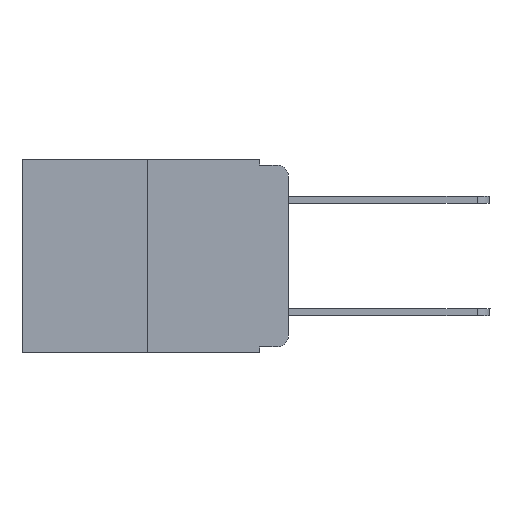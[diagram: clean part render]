
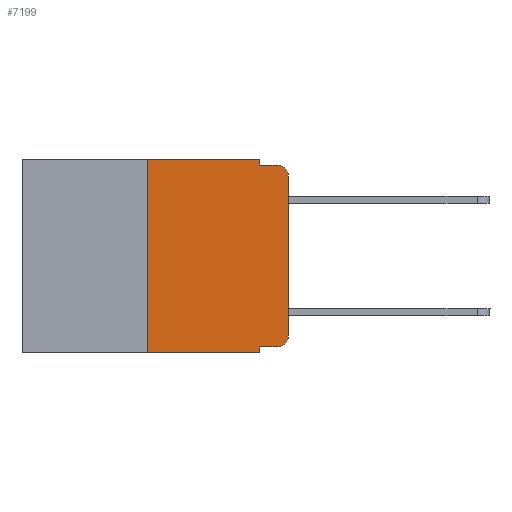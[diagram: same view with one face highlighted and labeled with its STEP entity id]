
A CAD part, left-side view. The second image highlights one B-rep face of the part: STEP entity #7199.
In plain terms, the highlighted planar face has unit normal (-1, 0, 0).
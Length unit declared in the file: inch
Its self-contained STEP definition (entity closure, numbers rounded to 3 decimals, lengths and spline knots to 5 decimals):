
#100 = CARTESIAN_POINT ( 'NONE',  ( 0., 0.25, 0. ) ) ;
#232 = VERTEX_POINT ( 'NONE', #6437 ) ;
#743 = DIRECTION ( 'NONE',  ( 0., 0., -1. ) ) ;
#809 = LINE ( 'NONE', #5505, #2120 ) ;
#894 = CARTESIAN_POINT ( 'NONE',  ( 0., 0.051, 0. ) ) ;
#1016 = DIRECTION ( 'NONE',  ( 0., 0., -1. ) ) ;
#1036 = CARTESIAN_POINT ( 'NONE',  ( 0., 0.051, 0. ) ) ;
#1127 = LINE ( 'NONE', #10622, #5782 ) ;
#1220 = AXIS2_PLACEMENT_3D ( 'NONE', #9701, #6009, #1016 ) ;
#1239 = DIRECTION ( 'NONE',  ( 0., 0., 1. ) ) ;
#1463 = VERTEX_POINT ( 'NONE', #8393 ) ;
#1633 = VECTOR ( 'NONE', #11658, 39.37008 ) ;
#1642 = CIRCLE ( 'NONE', #1220, 0.02 ) ;
#1655 = EDGE_CURVE ( 'NONE', #2808, #3309, #1127, .T. ) ;
#1686 = PLANE ( 'NONE',  #7245 ) ;
#1688 = ORIENTED_EDGE ( 'NONE', *, *, #10585, .F. ) ;
#1778 = LINE ( 'NONE', #8451, #8004 ) ;
#2067 = CARTESIAN_POINT ( 'NONE',  ( 0., 0., -0.313 ) ) ;
#2078 = LINE ( 'NONE', #9680, #12343 ) ;
#2120 = VECTOR ( 'NONE', #3590, 39.37008 ) ;
#2335 = EDGE_CURVE ( 'NONE', #8876, #6976, #4752, .T. ) ;
#2456 = VECTOR ( 'NONE', #6667, 39.37008 ) ;
#2649 = LINE ( 'NONE', #1036, #8716 ) ;
#2735 = EDGE_CURVE ( 'NONE', #232, #9243, #1778, .T. ) ;
#2808 = VERTEX_POINT ( 'NONE', #100 ) ;
#3199 = EDGE_LOOP ( 'NONE', ( #5355, #8519, #10112, #9112, #11165, #4226, #4914, #1688, #4359, #11659 ) ) ;
#3309 = VERTEX_POINT ( 'NONE', #894 ) ;
#3326 = VERTEX_POINT ( 'NONE', #12293 ) ;
#3590 = DIRECTION ( 'NONE',  ( 0., 0., 1. ) ) ;
#3822 = EDGE_CURVE ( 'NONE', #6976, #11323, #7746, .T. ) ;
#3920 = DIRECTION ( 'NONE',  ( 0., -1., 0. ) ) ;
#4150 = EDGE_CURVE ( 'NONE', #3309, #3326, #11232, .T. ) ;
#4226 = ORIENTED_EDGE ( 'NONE', *, *, #5027, .F. ) ;
#4359 = ORIENTED_EDGE ( 'NONE', *, *, #7975, .T. ) ;
#4653 = FACE_OUTER_BOUND ( 'NONE', #3199, .T. ) ;
#4752 = CIRCLE ( 'NONE', #5956, 0.02 ) ;
#4914 = ORIENTED_EDGE ( 'NONE', *, *, #2735, .T. ) ;
#5027 = EDGE_CURVE ( 'NONE', #232, #2808, #809, .T. ) ;
#5143 = EDGE_CURVE ( 'NONE', #3326, #9227, #2078, .T. ) ;
#5355 = ORIENTED_EDGE ( 'NONE', *, *, #3822, .T. ) ;
#5449 = CARTESIAN_POINT ( 'NONE',  ( 0., 0., -0.03 ) ) ;
#5505 = CARTESIAN_POINT ( 'NONE',  ( 0., 0.25, 0. ) ) ;
#5782 = VECTOR ( 'NONE', #3920, 39.37008 ) ;
#5956 = AXIS2_PLACEMENT_3D ( 'NONE', #12193, #9225, #9298 ) ;
#6009 = DIRECTION ( 'NONE',  ( -1., 0., 0. ) ) ;
#6099 = CARTESIAN_POINT ( 'NONE',  ( 0., 0.02, -0.333 ) ) ;
#6437 = CARTESIAN_POINT ( 'NONE',  ( 0., 0.25, -0.343 ) ) ;
#6590 = CARTESIAN_POINT ( 'NONE',  ( 0., 0.02, -0.01 ) ) ;
#6667 = DIRECTION ( 'NONE',  ( 0., 0., -1. ) ) ;
#6775 = CARTESIAN_POINT ( 'NONE',  ( 0., 0.051, -0.343 ) ) ;
#6832 = LINE ( 'NONE', #7903, #1633 ) ;
#6976 = VERTEX_POINT ( 'NONE', #2067 ) ;
#7199 = ADVANCED_FACE ( 'NONE', ( #4653 ), #1686, .F. ) ;
#7245 = AXIS2_PLACEMENT_3D ( 'NONE', #10225, #7418, #10351 ) ;
#7418 = DIRECTION ( 'NONE',  ( 1., 0., 0. ) ) ;
#7552 = CARTESIAN_POINT ( 'NONE',  ( 0., 0.051, 0. ) ) ;
#7746 = LINE ( 'NONE', #7861, #12371 ) ;
#7861 = CARTESIAN_POINT ( 'NONE',  ( 0., 0., 0. ) ) ;
#7903 = CARTESIAN_POINT ( 'NONE',  ( 0., 0.051, -0.333 ) ) ;
#7975 = EDGE_CURVE ( 'NONE', #1463, #8876, #6832, .T. ) ;
#8004 = VECTOR ( 'NONE', #12284, 39.37008 ) ;
#8393 = CARTESIAN_POINT ( 'NONE',  ( 0., 0.051, -0.333 ) ) ;
#8451 = CARTESIAN_POINT ( 'NONE',  ( 0., 0.473, -0.343 ) ) ;
#8453 = EDGE_CURVE ( 'NONE', #11323, #9227, #1642, .T. ) ;
#8519 = ORIENTED_EDGE ( 'NONE', *, *, #8453, .T. ) ;
#8716 = VECTOR ( 'NONE', #743, 39.37008 ) ;
#8876 = VERTEX_POINT ( 'NONE', #6099 ) ;
#9112 = ORIENTED_EDGE ( 'NONE', *, *, #4150, .F. ) ;
#9225 = DIRECTION ( 'NONE',  ( -1., 0., 0. ) ) ;
#9227 = VERTEX_POINT ( 'NONE', #6590 ) ;
#9243 = VERTEX_POINT ( 'NONE', #6775 ) ;
#9298 = DIRECTION ( 'NONE',  ( 0., 0., -1. ) ) ;
#9680 = CARTESIAN_POINT ( 'NONE',  ( 0., 0.051, -0.01 ) ) ;
#9701 = CARTESIAN_POINT ( 'NONE',  ( 0., 0.02, -0.03 ) ) ;
#10112 = ORIENTED_EDGE ( 'NONE', *, *, #5143, .F. ) ;
#10225 = CARTESIAN_POINT ( 'NONE',  ( 0., 0.473, 0. ) ) ;
#10351 = DIRECTION ( 'NONE',  ( 0., 0., -1. ) ) ;
#10585 = EDGE_CURVE ( 'NONE', #1463, #9243, #2649, .T. ) ;
#10622 = CARTESIAN_POINT ( 'NONE',  ( 0., 0.473, 0. ) ) ;
#11165 = ORIENTED_EDGE ( 'NONE', *, *, #1655, .F. ) ;
#11232 = LINE ( 'NONE', #7552, #2456 ) ;
#11323 = VERTEX_POINT ( 'NONE', #5449 ) ;
#11561 = DIRECTION ( 'NONE',  ( 0., -1., 0. ) ) ;
#11658 = DIRECTION ( 'NONE',  ( 0., -1., 0. ) ) ;
#11659 = ORIENTED_EDGE ( 'NONE', *, *, #2335, .T. ) ;
#12193 = CARTESIAN_POINT ( 'NONE',  ( 0., 0.02, -0.313 ) ) ;
#12284 = DIRECTION ( 'NONE',  ( 0., -1., 0. ) ) ;
#12293 = CARTESIAN_POINT ( 'NONE',  ( 0., 0.051, -0.01 ) ) ;
#12343 = VECTOR ( 'NONE', #11561, 39.37008 ) ;
#12371 = VECTOR ( 'NONE', #1239, 39.37008 ) ;
